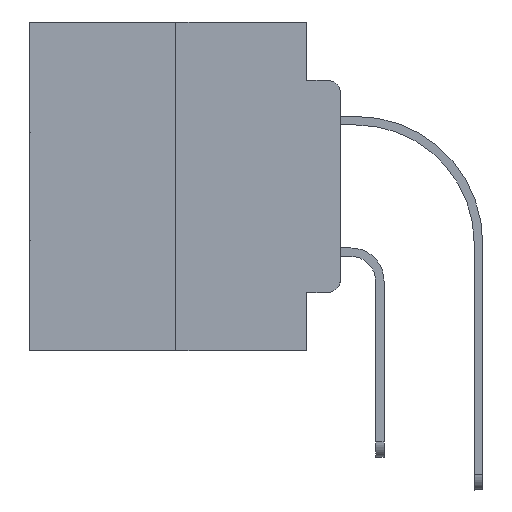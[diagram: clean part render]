
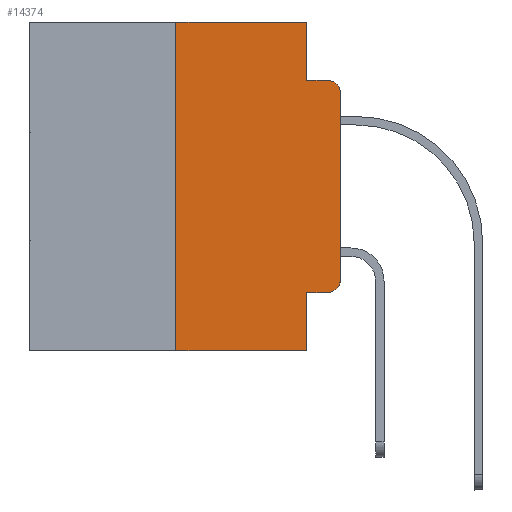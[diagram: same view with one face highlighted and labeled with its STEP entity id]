
A CAD part, left-side view. The second image highlights one B-rep face of the part: STEP entity #14374.
In plain terms, the highlighted planar face has unit normal (-1, 0, 0).
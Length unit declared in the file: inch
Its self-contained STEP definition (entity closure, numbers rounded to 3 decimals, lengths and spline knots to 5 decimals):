
#15 = LINE ( 'NONE', #17831, #17737 ) ;
#121 = CARTESIAN_POINT ( 'NONE',  ( 0., 0.02, -0.0885 ) ) ;
#821 = LINE ( 'NONE', #9736, #22765 ) ;
#864 = LINE ( 'NONE', #7883, #28108 ) ;
#1457 = VERTEX_POINT ( 'NONE', #25606 ) ;
#1633 = CARTESIAN_POINT ( 'NONE',  ( 0., 0.051, -0.0885 ) ) ;
#1666 = VERTEX_POINT ( 'NONE', #11855 ) ;
#2326 = EDGE_CURVE ( 'NONE', #1666, #8898, #864, .T. ) ;
#2481 = ORIENTED_EDGE ( 'NONE', *, *, #14581, .F. ) ;
#3231 = ORIENTED_EDGE ( 'NONE', *, *, #8212, .F. ) ;
#3674 = LINE ( 'NONE', #5879, #22386 ) ;
#4154 = ORIENTED_EDGE ( 'NONE', *, *, #9704, .F. ) ;
#4531 = LINE ( 'NONE', #26298, #19412 ) ;
#4622 = LINE ( 'NONE', #17916, #10638 ) ;
#4626 = CIRCLE ( 'NONE', #17233, 0.02 ) ;
#5731 = DIRECTION ( 'NONE',  ( -1., 0., 0. ) ) ;
#5879 = CARTESIAN_POINT ( 'NONE',  ( 0., 0.473, -0.5 ) ) ;
#5880 = DIRECTION ( 'NONE',  ( 0., 0., -1. ) ) ;
#6021 = DIRECTION ( 'NONE',  ( 0., -1., 0. ) ) ;
#6139 = DIRECTION ( 'NONE',  ( 0., -1., 0. ) ) ;
#6782 = DIRECTION ( 'NONE',  ( 0., 0., -1. ) ) ;
#7883 = CARTESIAN_POINT ( 'NONE',  ( 0., 0.051, -0.4115 ) ) ;
#8212 = EDGE_CURVE ( 'NONE', #27340, #26974, #4622, .T. ) ;
#8479 = EDGE_CURVE ( 'NONE', #1457, #27340, #821, .T. ) ;
#8898 = VERTEX_POINT ( 'NONE', #25470 ) ;
#9704 = EDGE_CURVE ( 'NONE', #26974, #21323, #12697, .T. ) ;
#9736 = CARTESIAN_POINT ( 'NONE',  ( 0., 0.473, 0. ) ) ;
#10113 = AXIS2_PLACEMENT_3D ( 'NONE', #14178, #28049, #23674 ) ;
#10171 = ORIENTED_EDGE ( 'NONE', *, *, #2326, .T. ) ;
#10202 = VERTEX_POINT ( 'NONE', #12385 ) ;
#10638 = VECTOR ( 'NONE', #24490, 39.37008 ) ;
#10735 = ORIENTED_EDGE ( 'NONE', *, *, #24885, .T. ) ;
#10951 = EDGE_CURVE ( 'NONE', #1666, #15166, #15681, .T. ) ;
#11550 = DIRECTION ( 'NONE',  ( 0., 0., 1. ) ) ;
#11855 = CARTESIAN_POINT ( 'NONE',  ( 0., 0.051, -0.4115 ) ) ;
#11861 = VECTOR ( 'NONE', #6782, 39.37008 ) ;
#12385 = CARTESIAN_POINT ( 'NONE',  ( 0., 0., -0.3915 ) ) ;
#12585 = PLANE ( 'NONE',  #26399 ) ;
#12697 = LINE ( 'NONE', #17232, #28363 ) ;
#12779 = EDGE_CURVE ( 'NONE', #20268, #21323, #21302, .T. ) ;
#14178 = CARTESIAN_POINT ( 'NONE',  ( 0., 0.02, -0.1085 ) ) ;
#14374 = ADVANCED_FACE ( 'NONE', ( #19023 ), #12585, .F. ) ;
#14581 = EDGE_CURVE ( 'NONE', #20986, #1457, #4531, .T. ) ;
#14782 = CARTESIAN_POINT ( 'NONE',  ( 0., 0.473, 0. ) ) ;
#15166 = VERTEX_POINT ( 'NONE', #22605 ) ;
#15212 = DIRECTION ( 'NONE',  ( 0., 0., 1. ) ) ;
#15626 = EDGE_CURVE ( 'NONE', #8898, #10202, #4626, .T. ) ;
#15681 = LINE ( 'NONE', #17869, #11861 ) ;
#15817 = ORIENTED_EDGE ( 'NONE', *, *, #8479, .F. ) ;
#16352 = DIRECTION ( 'NONE',  ( 0., -1., 0. ) ) ;
#16833 = DIRECTION ( 'NONE',  ( 0., 0., -1. ) ) ;
#16969 = DIRECTION ( 'NONE',  ( 1., 0., 0. ) ) ;
#17043 = CARTESIAN_POINT ( 'NONE',  ( 0., 0., -0.1085 ) ) ;
#17088 = CARTESIAN_POINT ( 'NONE',  ( 0., 0.25, -0.5 ) ) ;
#17232 = CARTESIAN_POINT ( 'NONE',  ( 0., 0.051, -0.0885 ) ) ;
#17233 = AXIS2_PLACEMENT_3D ( 'NONE', #28504, #5731, #16833 ) ;
#17737 = VECTOR ( 'NONE', #11550, 39.37008 ) ;
#17831 = CARTESIAN_POINT ( 'NONE',  ( 0., 0., 0. ) ) ;
#17869 = CARTESIAN_POINT ( 'NONE',  ( 0., 0.051, 0. ) ) ;
#17916 = CARTESIAN_POINT ( 'NONE',  ( 0., 0.051, 0. ) ) ;
#18448 = ORIENTED_EDGE ( 'NONE', *, *, #20812, .T. ) ;
#19023 = FACE_OUTER_BOUND ( 'NONE', #19388, .T. ) ;
#19388 = EDGE_LOOP ( 'NONE', ( #18448, #28802, #4154, #3231, #15817, #2481, #10735, #19880, #10171, #26889 ) ) ;
#19412 = VECTOR ( 'NONE', #15212, 39.37008 ) ;
#19880 = ORIENTED_EDGE ( 'NONE', *, *, #10951, .F. ) ;
#20268 = VERTEX_POINT ( 'NONE', #17043 ) ;
#20812 = EDGE_CURVE ( 'NONE', #10202, #20268, #15, .T. ) ;
#20986 = VERTEX_POINT ( 'NONE', #17088 ) ;
#21302 = CIRCLE ( 'NONE', #10113, 0.02 ) ;
#21323 = VERTEX_POINT ( 'NONE', #121 ) ;
#22386 = VECTOR ( 'NONE', #6021, 39.37008 ) ;
#22605 = CARTESIAN_POINT ( 'NONE',  ( 0., 0.051, -0.5 ) ) ;
#22765 = VECTOR ( 'NONE', #28115, 39.37008 ) ;
#23674 = DIRECTION ( 'NONE',  ( 0., 0., -1. ) ) ;
#24490 = DIRECTION ( 'NONE',  ( 0., 0., -1. ) ) ;
#24885 = EDGE_CURVE ( 'NONE', #20986, #15166, #3674, .T. ) ;
#25470 = CARTESIAN_POINT ( 'NONE',  ( 0., 0.02, -0.4115 ) ) ;
#25606 = CARTESIAN_POINT ( 'NONE',  ( 0., 0.25, 0. ) ) ;
#26298 = CARTESIAN_POINT ( 'NONE',  ( 0., 0.25, 0. ) ) ;
#26399 = AXIS2_PLACEMENT_3D ( 'NONE', #14782, #16969, #5880 ) ;
#26889 = ORIENTED_EDGE ( 'NONE', *, *, #15626, .T. ) ;
#26974 = VERTEX_POINT ( 'NONE', #1633 ) ;
#27340 = VERTEX_POINT ( 'NONE', #28472 ) ;
#28049 = DIRECTION ( 'NONE',  ( -1., 0., 0. ) ) ;
#28108 = VECTOR ( 'NONE', #16352, 39.37008 ) ;
#28115 = DIRECTION ( 'NONE',  ( 0., -1., 0. ) ) ;
#28363 = VECTOR ( 'NONE', #6139, 39.37008 ) ;
#28472 = CARTESIAN_POINT ( 'NONE',  ( 0., 0.051, 0. ) ) ;
#28504 = CARTESIAN_POINT ( 'NONE',  ( 0., 0.02, -0.3915 ) ) ;
#28802 = ORIENTED_EDGE ( 'NONE', *, *, #12779, .T. ) ;
